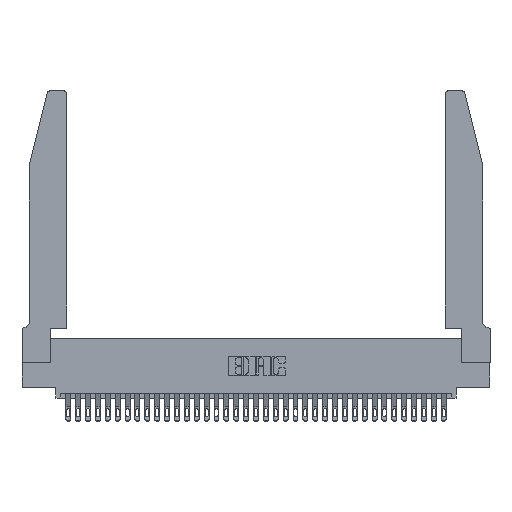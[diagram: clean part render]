
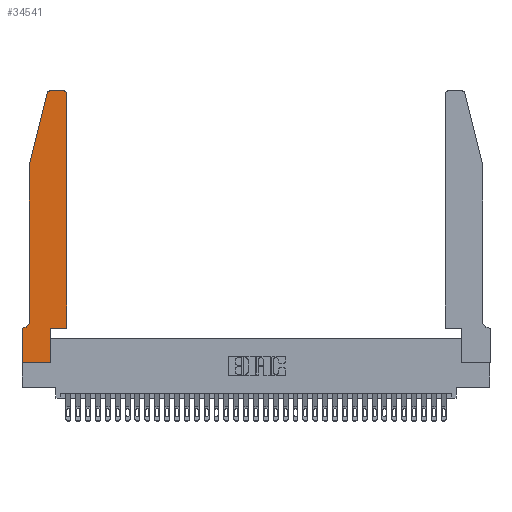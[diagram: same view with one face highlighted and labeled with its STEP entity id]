
A CAD part, top view. The second image highlights one B-rep face of the part: STEP entity #34541.
In plain terms, the highlighted planar face has unit normal (0, 0, 1).
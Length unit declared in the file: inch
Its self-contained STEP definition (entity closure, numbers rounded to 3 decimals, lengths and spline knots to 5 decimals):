
#265 = ORIENTED_EDGE ( 'NONE', *, *, #5840, .T. ) ;
#271 = DIRECTION ( 'NONE',  ( 0., -1., 0. ) ) ;
#610 = CARTESIAN_POINT ( 'NONE',  ( 0.284, 2.72, 0.37 ) ) ;
#993 = EDGE_CURVE ( 'NONE', #30638, #33720, #24504, .T. ) ;
#1740 = DIRECTION ( 'NONE',  ( -1., 0., 0. ) ) ;
#2220 = CARTESIAN_POINT ( 'NONE',  ( 0.4505, 0.35, 0.37 ) ) ;
#3532 = DIRECTION ( 'NONE',  ( 1., 0., 0. ) ) ;
#3800 = LINE ( 'NONE', #2220, #17908 ) ;
#4087 = EDGE_CURVE ( 'NONE', #31681, #32282, #24715, .T. ) ;
#4146 = DIRECTION ( 'NONE',  ( 0., 1., 0. ) ) ;
#4166 = CARTESIAN_POINT ( 'NONE',  ( 0.0055, 0.35, 0.37 ) ) ;
#4832 = CARTESIAN_POINT ( 'NONE',  ( 0.0055, 0.42, 0.37 ) ) ;
#5840 = EDGE_CURVE ( 'NONE', #29343, #34456, #14464, .T. ) ;
#6330 = VECTOR ( 'NONE', #1740, 39.37008 ) ;
#6365 = DIRECTION ( 'NONE',  ( -1., 0., 0. ) ) ;
#6851 = CARTESIAN_POINT ( 'NONE',  ( 0., 0.35, 0.37 ) ) ;
#7293 = AXIS2_PLACEMENT_3D ( 'NONE', #6851, #15317, #34713 ) ;
#7669 = DIRECTION ( 'NONE',  ( -1., 0., 0. ) ) ;
#7820 = CARTESIAN_POINT ( 'NONE',  ( 0.0755, 2., 0.37 ) ) ;
#7896 = VERTEX_POINT ( 'NONE', #23315 ) ;
#8397 = ORIENTED_EDGE ( 'NONE', *, *, #4087, .T. ) ;
#8519 = DIRECTION ( 'NONE',  ( 0., 0., 1. ) ) ;
#9203 = CIRCLE ( 'NONE', #11333, 0.03 ) ;
#9617 = VECTOR ( 'NONE', #25536, 39.37008 ) ;
#10323 = CARTESIAN_POINT ( 'NONE',  ( 0.2605, 2.75, 0.37 ) ) ;
#10510 = EDGE_CURVE ( 'NONE', #25975, #31681, #16013, .T. ) ;
#10963 = ORIENTED_EDGE ( 'NONE', *, *, #18483, .T. ) ;
#11333 = AXIS2_PLACEMENT_3D ( 'NONE', #25277, #8519, #28043 ) ;
#11453 = CARTESIAN_POINT ( 'NONE',  ( 0., 0., 0.37 ) ) ;
#11688 = CARTESIAN_POINT ( 'NONE',  ( 0., 0., 0.37 ) ) ;
#12437 = CIRCLE ( 'NONE', #20194, 0.03 ) ;
#13366 = VECTOR ( 'NONE', #4146, 39.37008 ) ;
#13769 = VECTOR ( 'NONE', #6365, 39.37008 ) ;
#13773 = CARTESIAN_POINT ( 'NONE',  ( 0.2865, 0.35, 0.37 ) ) ;
#14142 = DIRECTION ( 'NONE',  ( -0.239, -0.971, 0. ) ) ;
#14262 = EDGE_CURVE ( 'NONE', #34456, #30638, #28174, .T. ) ;
#14438 = CARTESIAN_POINT ( 'NONE',  ( 0.0755, 2., 0.37 ) ) ;
#14464 = LINE ( 'NONE', #29396, #21646 ) ;
#14633 = LINE ( 'NONE', #14724, #13769 ) ;
#14724 = CARTESIAN_POINT ( 'NONE',  ( 0.0755, 0.35, 0.37 ) ) ;
#15317 = DIRECTION ( 'NONE',  ( 0., 0., 1. ) ) ;
#15820 = CARTESIAN_POINT ( 'NONE',  ( 0.4205, 2.75, 0.37 ) ) ;
#16013 = LINE ( 'NONE', #14438, #22589 ) ;
#17118 = ORIENTED_EDGE ( 'NONE', *, *, #14262, .T. ) ;
#17615 = ORIENTED_EDGE ( 'NONE', *, *, #21881, .T. ) ;
#17908 = VECTOR ( 'NONE', #35671, 39.37008 ) ;
#17951 = EDGE_CURVE ( 'NONE', #30172, #29343, #33528, .T. ) ;
#18385 = VERTEX_POINT ( 'NONE', #15820 ) ;
#18483 = EDGE_CURVE ( 'NONE', #33720, #20244, #3800, .T. ) ;
#20149 = ORIENTED_EDGE ( 'NONE', *, *, #21483, .T. ) ;
#20194 = AXIS2_PLACEMENT_3D ( 'NONE', #610, #20387, #3532 ) ;
#20244 = VERTEX_POINT ( 'NONE', #27700 ) ;
#20333 = FACE_OUTER_BOUND ( 'NONE', #20986, .T. ) ;
#20382 = LINE ( 'NONE', #10323, #6330 ) ;
#20387 = DIRECTION ( 'NONE',  ( 0., 0., 1. ) ) ;
#20983 = CARTESIAN_POINT ( 'NONE',  ( 0.2865, 0.35, 0.37 ) ) ;
#20986 = EDGE_LOOP ( 'NONE', ( #32121, #20149, #17615, #21090, #8397, #24135, #33192, #265, #17118, #33568, #10963, #24522 ) ) ;
#21090 = ORIENTED_EDGE ( 'NONE', *, *, #10510, .T. ) ;
#21204 = EDGE_CURVE ( 'NONE', #32282, #30172, #14633, .T. ) ;
#21483 = EDGE_CURVE ( 'NONE', #7896, #30089, #12437, .T. ) ;
#21609 = AXIS2_PLACEMENT_3D ( 'NONE', #4832, #24454, #7669 ) ;
#21646 = VECTOR ( 'NONE', #23858, 39.37008 ) ;
#21881 = EDGE_CURVE ( 'NONE', #30089, #25975, #34533, .T. ) ;
#22454 = CARTESIAN_POINT ( 'NONE',  ( 0.0755, 2., 0.37 ) ) ;
#22589 = VECTOR ( 'NONE', #271, 39.37008 ) ;
#22975 = CARTESIAN_POINT ( 'NONE',  ( 0.4505, 0.35, 0.37 ) ) ;
#23315 = CARTESIAN_POINT ( 'NONE',  ( 0.284, 2.75, 0.37 ) ) ;
#23858 = DIRECTION ( 'NONE',  ( 1., 0., 0. ) ) ;
#24135 = ORIENTED_EDGE ( 'NONE', *, *, #21204, .T. ) ;
#24454 = DIRECTION ( 'NONE',  ( 0., 0., -1. ) ) ;
#24504 = LINE ( 'NONE', #28309, #9617 ) ;
#24522 = ORIENTED_EDGE ( 'NONE', *, *, #24850, .T. ) ;
#24715 = CIRCLE ( 'NONE', #21609, 0.07 ) ;
#24850 = EDGE_CURVE ( 'NONE', #20244, #18385, #9203, .T. ) ;
#25277 = CARTESIAN_POINT ( 'NONE',  ( 0.4205, 2.72, 0.37 ) ) ;
#25536 = DIRECTION ( 'NONE',  ( 1., 0., 0. ) ) ;
#25975 = VERTEX_POINT ( 'NONE', #7820 ) ;
#27081 = VECTOR ( 'NONE', #28155, 39.37008 ) ;
#27635 = EDGE_CURVE ( 'NONE', #18385, #7896, #20382, .T. ) ;
#27700 = CARTESIAN_POINT ( 'NONE',  ( 0.4505, 2.72, 0.37 ) ) ;
#28043 = DIRECTION ( 'NONE',  ( 1., 0., 0. ) ) ;
#28155 = DIRECTION ( 'NONE',  ( 0., -1., 0. ) ) ;
#28174 = LINE ( 'NONE', #20983, #13366 ) ;
#28309 = CARTESIAN_POINT ( 'NONE',  ( 0.4505, 0.35, 0.37 ) ) ;
#29343 = VERTEX_POINT ( 'NONE', #11688 ) ;
#29396 = CARTESIAN_POINT ( 'NONE',  ( 0., 0., 0.37 ) ) ;
#30089 = VERTEX_POINT ( 'NONE', #33579 ) ;
#30172 = VERTEX_POINT ( 'NONE', #31268 ) ;
#30638 = VERTEX_POINT ( 'NONE', #13773 ) ;
#31268 = CARTESIAN_POINT ( 'NONE',  ( 0., 0.35, 0.37 ) ) ;
#31594 = CARTESIAN_POINT ( 'NONE',  ( 0.2865, 0., 0.37 ) ) ;
#31681 = VERTEX_POINT ( 'NONE', #34680 ) ;
#31950 = PLANE ( 'NONE',  #7293 ) ;
#32121 = ORIENTED_EDGE ( 'NONE', *, *, #27635, .T. ) ;
#32282 = VERTEX_POINT ( 'NONE', #4166 ) ;
#33192 = ORIENTED_EDGE ( 'NONE', *, *, #17951, .T. ) ;
#33528 = LINE ( 'NONE', #11453, #27081 ) ;
#33568 = ORIENTED_EDGE ( 'NONE', *, *, #993, .T. ) ;
#33579 = CARTESIAN_POINT ( 'NONE',  ( 0.25487, 2.72718, 0.37 ) ) ;
#33677 = VECTOR ( 'NONE', #14142, 39.37008 ) ;
#33720 = VERTEX_POINT ( 'NONE', #22975 ) ;
#34456 = VERTEX_POINT ( 'NONE', #31594 ) ;
#34533 = LINE ( 'NONE', #22454, #33677 ) ;
#34541 = ADVANCED_FACE ( 'NONE', ( #20333 ), #31950, .T. ) ;
#34680 = CARTESIAN_POINT ( 'NONE',  ( 0.0755, 0.42, 0.37 ) ) ;
#34713 = DIRECTION ( 'NONE',  ( 1., 0., 0. ) ) ;
#35671 = DIRECTION ( 'NONE',  ( 0., 1., 0. ) ) ;
